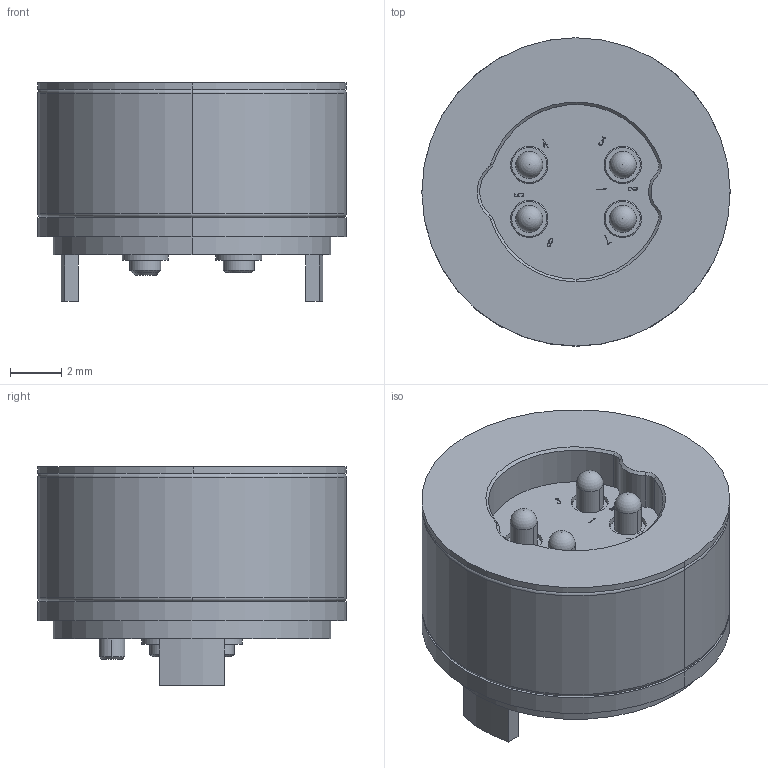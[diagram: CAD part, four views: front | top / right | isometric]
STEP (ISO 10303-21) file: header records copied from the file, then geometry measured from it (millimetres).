
FILE_DESCRIPTION (( 'STEP AP203' ), '1' );
FILE_NAME ('685-A04222A01E1.STEP', '2023-02-03T17:09:59', ( 'Magnum' ), ( '' ), 'SwSTEP 2.0', 'SolidWorks 2020', '' );
FILE_SCHEMA (( 'CONFIG_CONTROL_DESIGN' ));
Length unit declared in the file: millimetre
Products named in the file (1): 685-A04222A01E1
Bounding box: 12 x 12 x 8.5 mm (x, y, z)
Surface area: 788.5 mm2 (no closed solid volume)
Topology: 0 solids, 8 shells, 333 faces, 837 edges, 546 vertices
Faces by surface type: plane 140, cylinder 116, bspline 34, cone 29, sphere 8, torus 6
Entity records: 11938 total; most frequent: CARTESIAN_POINT 4013, ORIENTED_EDGE 1644, DIRECTION 1596, EDGE_CURVE 823, AXIS2_PLACEMENT_3D 585, VERTEX_POINT 538, LINE 426, VECTOR 426
